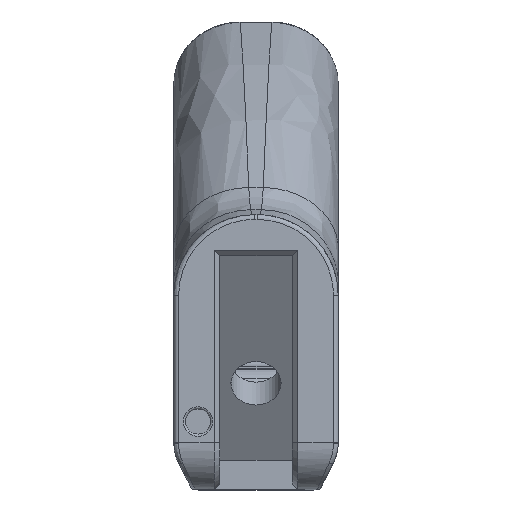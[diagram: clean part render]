
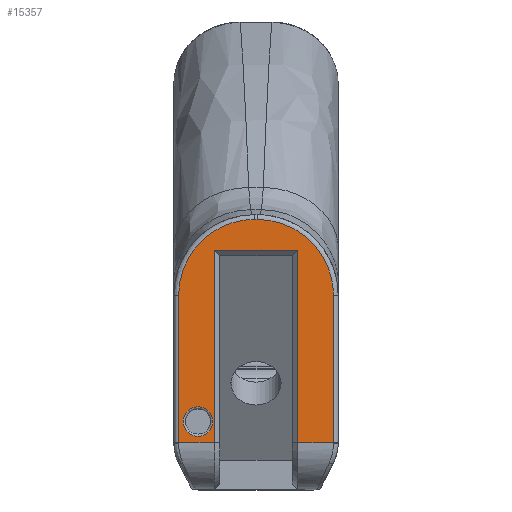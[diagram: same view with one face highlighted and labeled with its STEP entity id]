
A CAD part, top view. The second image highlights one B-rep face of the part: STEP entity #15357.
In plain terms, the highlighted planar face has unit normal (0, 0, 1).
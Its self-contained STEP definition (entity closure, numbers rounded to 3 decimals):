
#165=FACE_BOUND('',#3797,.T.);
#316=PLANE('',#16426);
#785=LINE('',#38487,#1458);
#788=LINE('',#38691,#1461);
#814=LINE('',#39943,#1487);
#860=LINE('',#41136,#1533);
#867=LINE('',#41153,#1540);
#872=LINE('',#41165,#1545);
#902=LINE('',#42286,#1575);
#904=LINE('',#42328,#1577);
#1458=VECTOR('',#18137,10.);
#1461=VECTOR('',#18164,10.);
#1487=VECTOR('',#18240,10.);
#1533=VECTOR('',#18544,10.);
#1540=VECTOR('',#18561,10.);
#1545=VECTOR('',#18574,10.);
#1575=VECTOR('',#18688,10.);
#1577=VECTOR('',#18696,10.);
#2839=FACE_OUTER_BOUND('',#3796,.T.);
#3796=EDGE_LOOP('',(#13751,#13752,#13753,#13754,#13755,#13756,#13757,#13758,
#13759,#13760));
#3797=EDGE_LOOP('',(#13761));
#4559=B_SPLINE_CURVE_WITH_KNOTS('',3,(#38527,#38528,#38529,#38530,#38531,
#38532),.UNSPECIFIED.,.F.,.F.,(4,1,1,4),(0.,0.696,1.16,
1.623),.UNSPECIFIED.);
#4690=B_SPLINE_CURVE_WITH_KNOTS('',3,(#42321,#42322,#42323,#42324,#42325,
#42326),.UNSPECIFIED.,.F.,.F.,(4,1,1,4),(0.,0.464,0.928,
1.623),.UNSPECIFIED.);
#5409=CIRCLE('',#16427,2.);
#6477=VERTEX_POINT('',#38483);
#6478=VERTEX_POINT('',#38485);
#6480=VERTEX_POINT('',#38525);
#6491=VERTEX_POINT('',#38690);
#6534=VERTEX_POINT('',#39941);
#6588=VERTEX_POINT('',#41133);
#6589=VERTEX_POINT('',#41135);
#6597=VERTEX_POINT('',#41164);
#6654=VERTEX_POINT('',#42285);
#6655=VERTEX_POINT('',#42319);
#6849=VERTEX_POINT('',#45545);
#8479=EDGE_CURVE('',#6478,#6477,#785,.T.);
#8482=EDGE_CURVE('',#6480,#6478,#4559,.T.);
#8499=EDGE_CURVE('',#6477,#6491,#788,.T.);
#8583=EDGE_CURVE('',#6491,#6534,#814,.T.);
#8715=EDGE_CURVE('',#6588,#6589,#860,.T.);
#8724=EDGE_CURVE('',#6534,#6588,#867,.T.);
#8730=EDGE_CURVE('',#6597,#6589,#872,.T.);
#8840=EDGE_CURVE('',#6597,#6654,#902,.T.);
#8844=EDGE_CURVE('',#6654,#6655,#4690,.T.);
#8845=EDGE_CURVE('',#6655,#6480,#904,.T.);
#9177=EDGE_CURVE('',#6849,#6849,#5409,.T.);
#13751=ORIENTED_EDGE('',*,*,#8845,.F.);
#13752=ORIENTED_EDGE('',*,*,#8844,.F.);
#13753=ORIENTED_EDGE('',*,*,#8840,.F.);
#13754=ORIENTED_EDGE('',*,*,#8730,.T.);
#13755=ORIENTED_EDGE('',*,*,#8715,.F.);
#13756=ORIENTED_EDGE('',*,*,#8724,.F.);
#13757=ORIENTED_EDGE('',*,*,#8583,.F.);
#13758=ORIENTED_EDGE('',*,*,#8499,.F.);
#13759=ORIENTED_EDGE('',*,*,#8479,.F.);
#13760=ORIENTED_EDGE('',*,*,#8482,.F.);
#13761=ORIENTED_EDGE('',*,*,#9177,.F.);
#15357=ADVANCED_FACE('',(#2839,#165),#316,.T.);
#16426=AXIS2_PLACEMENT_3D('',#45544,#19137,#19138);
#16427=AXIS2_PLACEMENT_3D('',#45546,#19139,#19140);
#18137=DIRECTION('',(0.,-1.,0.));
#18164=DIRECTION('',(-1.,0.,0.));
#18240=DIRECTION('',(0.,1.,0.));
#18544=DIRECTION('',(0.,-1.,0.));
#18561=DIRECTION('',(-1.,0.,0.));
#18574=DIRECTION('',(1.,0.,0.));
#18688=DIRECTION('',(0.,1.,0.));
#18696=DIRECTION('',(1.,0.,0.));
#19137=DIRECTION('center_axis',(0.,0.,
1.));
#19138=DIRECTION('ref_axis',(0.,-1.,0.));
#19139=DIRECTION('center_axis',(0.,0.,
1.));
#19140=DIRECTION('ref_axis',(1.,0.,0.));
#38483=CARTESIAN_POINT('',(34.595,-143.468,28.406));
#38485=CARTESIAN_POINT('',(34.595,-123.457,28.406));
#38487=CARTESIAN_POINT('',(34.595,-40.367,28.406));
#38525=CARTESIAN_POINT('',(24.26,-113.122,28.406));
#38527=CARTESIAN_POINT('Ctrl Pts',(24.26,-113.122,28.406));
#38528=CARTESIAN_POINT('Ctrl Pts',(26.579,-113.122,28.406));
#38529=CARTESIAN_POINT('Ctrl Pts',(30.43,-114.477,28.406));
#38530=CARTESIAN_POINT('Ctrl Pts',(33.888,-118.824,28.406));
#38531=CARTESIAN_POINT('Ctrl Pts',(34.595,-121.911,28.406));
#38532=CARTESIAN_POINT('Ctrl Pts',(34.595,-123.457,28.406));
#38690=CARTESIAN_POINT('',(29.746,-143.468,28.406));
#38691=CARTESIAN_POINT('',(19.207,-143.468,28.406));
#39941=CARTESIAN_POINT('',(29.746,-117.318,28.406));
#39943=CARTESIAN_POINT('',(29.746,-114.618,28.406));
#41133=CARTESIAN_POINT('',(18.417,-117.318,28.406));
#41135=CARTESIAN_POINT('',(18.417,-143.468,28.406));
#41136=CARTESIAN_POINT('',(18.417,-114.618,28.406));
#41153=CARTESIAN_POINT('',(24.173,-117.318,28.406));
#41164=CARTESIAN_POINT('',(13.568,-143.468,28.406));
#41165=CARTESIAN_POINT('',(28.956,-143.468,28.406));
#42285=CARTESIAN_POINT('',(13.568,-123.457,28.406));
#42286=CARTESIAN_POINT('',(13.568,-40.367,28.406));
#42319=CARTESIAN_POINT('',(23.903,-113.122,28.406));
#42321=CARTESIAN_POINT('Ctrl Pts',(13.568,-123.457,28.406));
#42322=CARTESIAN_POINT('Ctrl Pts',(13.568,-121.911,28.406));
#42323=CARTESIAN_POINT('Ctrl Pts',(14.275,-118.824,28.406));
#42324=CARTESIAN_POINT('Ctrl Pts',(17.732,-114.477,28.406));
#42325=CARTESIAN_POINT('Ctrl Pts',(21.584,-113.122,28.406));
#42326=CARTESIAN_POINT('Ctrl Pts',(23.903,-113.122,28.406));
#42328=CARTESIAN_POINT('',(27.226,-113.122,28.406));
#45544=CARTESIAN_POINT('Origin',(19.207,-112.624,28.406));
#45545=CARTESIAN_POINT('',(18.205,-140.572,28.406));
#45546=CARTESIAN_POINT('Origin',(16.205,-140.572,28.406));
